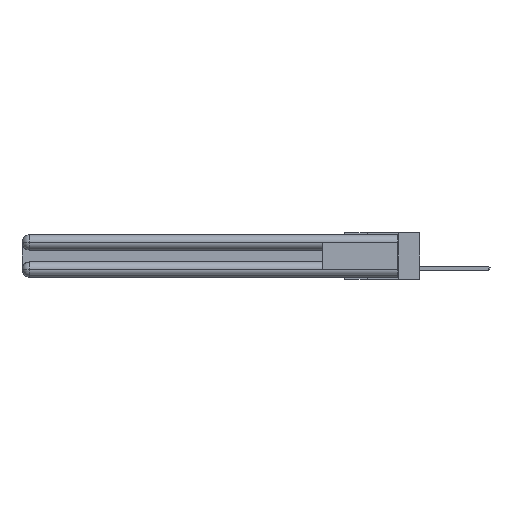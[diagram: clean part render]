
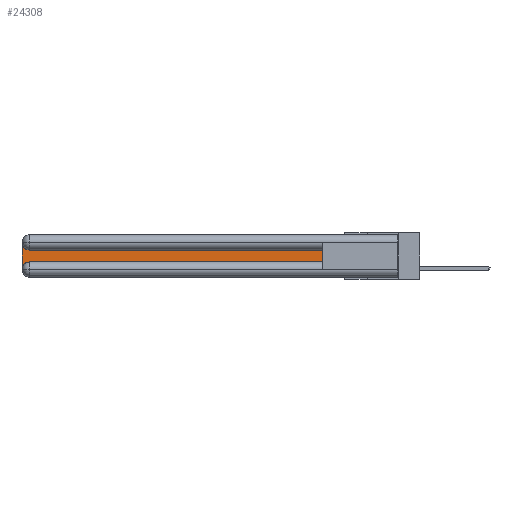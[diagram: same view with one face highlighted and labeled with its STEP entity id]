
A CAD part, left-side view. The second image highlights one B-rep face of the part: STEP entity #24308.
In plain terms, the highlighted planar face has unit normal (-1, 0, 0).
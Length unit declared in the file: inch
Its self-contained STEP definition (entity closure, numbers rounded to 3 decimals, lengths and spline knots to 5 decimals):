
#260 = VERTEX_POINT ( 'NONE', #10372 ) ;
#416 = VECTOR ( 'NONE', #24607, 39.37008 ) ;
#431 = EDGE_CURVE ( 'NONE', #11360, #17849, #19287, .T. ) ;
#956 = CARTESIAN_POINT ( 'NONE',  ( 0.075, 0.6, -0.1225 ) ) ;
#1255 = DIRECTION ( 'NONE',  ( 0., 0., -1. ) ) ;
#1478 = DIRECTION ( 'NONE',  ( 1., 0., 0. ) ) ;
#1692 = EDGE_CURVE ( 'NONE', #260, #10715, #15870, .T. ) ;
#1874 = CARTESIAN_POINT ( 'NONE',  ( 0.075, 2.94, -0.1225 ) ) ;
#1966 = VECTOR ( 'NONE', #23150, 39.37008 ) ;
#2623 = CARTESIAN_POINT ( 'NONE',  ( 0.075, 0.6, -0.2175 ) ) ;
#2972 = AXIS2_PLACEMENT_3D ( 'NONE', #3099, #18491, #13332 ) ;
#3099 = CARTESIAN_POINT ( 'NONE',  ( 0.075, 2.94, -0.0625 ) ) ;
#5280 = LINE ( 'NONE', #10180, #1966 ) ;
#6727 = VERTEX_POINT ( 'NONE', #14633 ) ;
#7400 = AXIS2_PLACEMENT_3D ( 'NONE', #11599, #1478, #1255 ) ;
#7594 = DIRECTION ( 'NONE',  ( 0., 0., 1. ) ) ;
#9144 = ORIENTED_EDGE ( 'NONE', *, *, #33773, .T. ) ;
#9400 = ORIENTED_EDGE ( 'NONE', *, *, #18768, .T. ) ;
#10180 = CARTESIAN_POINT ( 'NONE',  ( 0.075, 3., -0.2175 ) ) ;
#10227 = VECTOR ( 'NONE', #7594, 39.37008 ) ;
#10372 = CARTESIAN_POINT ( 'NONE',  ( 0.075, 2.94, -0.2175 ) ) ;
#10715 = VERTEX_POINT ( 'NONE', #27599 ) ;
#11360 = VERTEX_POINT ( 'NONE', #1874 ) ;
#11599 = CARTESIAN_POINT ( 'NONE',  ( 0.075, 3., -0.1225 ) ) ;
#12987 = EDGE_CURVE ( 'NONE', #33298, #11360, #21420, .T. ) ;
#13157 = CARTESIAN_POINT ( 'NONE',  ( 0.075, 3., -0.0625 ) ) ;
#13332 = DIRECTION ( 'NONE',  ( 0., 0., -1. ) ) ;
#14272 = ORIENTED_EDGE ( 'NONE', *, *, #12987, .T. ) ;
#14633 = CARTESIAN_POINT ( 'NONE',  ( 0.075, 3., -0.2775 ) ) ;
#14812 = DIRECTION ( 'NONE',  ( 1., 0., 0. ) ) ;
#15870 = LINE ( 'NONE', #21477, #26168 ) ;
#16679 = AXIS2_PLACEMENT_3D ( 'NONE', #25501, #14812, #20234 ) ;
#17332 = FACE_OUTER_BOUND ( 'NONE', #27949, .T. ) ;
#17849 = VERTEX_POINT ( 'NONE', #13157 ) ;
#18036 = LINE ( 'NONE', #2623, #10227 ) ;
#18491 = DIRECTION ( 'NONE',  ( 1., 0., 0. ) ) ;
#18768 = EDGE_CURVE ( 'NONE', #10715, #33298, #18036, .T. ) ;
#19287 = CIRCLE ( 'NONE', #2972, 0.06 ) ;
#19583 = CIRCLE ( 'NONE', #16679, 0.06 ) ;
#20234 = DIRECTION ( 'NONE',  ( 0., 0., -1. ) ) ;
#21420 = LINE ( 'NONE', #956, #416 ) ;
#21477 = CARTESIAN_POINT ( 'NONE',  ( 0.075, 0.6, -0.2175 ) ) ;
#23150 = DIRECTION ( 'NONE',  ( 0., 0., -1. ) ) ;
#24088 = DIRECTION ( 'NONE',  ( 0., -1., 0. ) ) ;
#24308 = ADVANCED_FACE ( 'NONE', ( #17332 ), #30078, .F. ) ;
#24607 = DIRECTION ( 'NONE',  ( 0., 1., 0. ) ) ;
#24997 = CARTESIAN_POINT ( 'NONE',  ( 0.075, 0.6, -0.1225 ) ) ;
#25501 = CARTESIAN_POINT ( 'NONE',  ( 0.075, 2.94, -0.2775 ) ) ;
#25667 = ORIENTED_EDGE ( 'NONE', *, *, #431, .T. ) ;
#25786 = ORIENTED_EDGE ( 'NONE', *, *, #27615, .T. ) ;
#26168 = VECTOR ( 'NONE', #24088, 39.37008 ) ;
#27599 = CARTESIAN_POINT ( 'NONE',  ( 0.075, 0.6, -0.2175 ) ) ;
#27615 = EDGE_CURVE ( 'NONE', #6727, #260, #19583, .T. ) ;
#27949 = EDGE_LOOP ( 'NONE', ( #14272, #25667, #9144, #25786, #32991, #9400 ) ) ;
#30078 = PLANE ( 'NONE',  #7400 ) ;
#32991 = ORIENTED_EDGE ( 'NONE', *, *, #1692, .T. ) ;
#33298 = VERTEX_POINT ( 'NONE', #24997 ) ;
#33773 = EDGE_CURVE ( 'NONE', #17849, #6727, #5280, .T. ) ;
